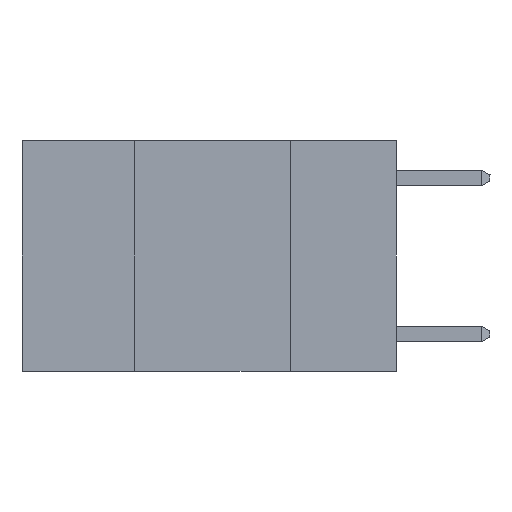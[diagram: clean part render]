
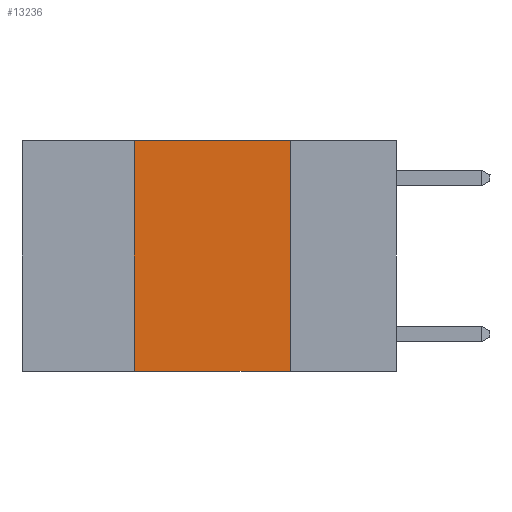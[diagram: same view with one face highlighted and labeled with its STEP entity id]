
A CAD part, left-side view. The second image highlights one B-rep face of the part: STEP entity #13236.
In plain terms, the highlighted planar face has unit normal (-1, 0, 0).
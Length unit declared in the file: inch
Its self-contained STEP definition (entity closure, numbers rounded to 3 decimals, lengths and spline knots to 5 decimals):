
#1128 = ORIENTED_EDGE ( 'NONE', *, *, #13991, .T. ) ;
#3027 = LINE ( 'NONE', #6565, #6303 ) ;
#3278 = EDGE_CURVE ( 'NONE', #15691, #15222, #6163, .T. ) ;
#3468 = PLANE ( 'NONE',  #9827 ) ;
#3547 = CARTESIAN_POINT ( 'NONE',  ( 0., 0.17, 0. ) ) ;
#3692 = LINE ( 'NONE', #3547, #11757 ) ;
#4470 = CARTESIAN_POINT ( 'NONE',  ( 0., 0.6, 0. ) ) ;
#6163 = LINE ( 'NONE', #4470, #9892 ) ;
#6303 = VECTOR ( 'NONE', #9366, 39.37008 ) ;
#6565 = CARTESIAN_POINT ( 'NONE',  ( 0., 0.6, -0.37 ) ) ;
#7215 = ORIENTED_EDGE ( 'NONE', *, *, #8718, .F. ) ;
#7657 = DIRECTION ( 'NONE',  ( 1., 0., 0. ) ) ;
#8599 = DIRECTION ( 'NONE',  ( 0., 0., 1. ) ) ;
#8718 = EDGE_CURVE ( 'NONE', #14443, #15691, #10187, .T. ) ;
#9366 = DIRECTION ( 'NONE',  ( 0., -1., 0. ) ) ;
#9404 = ORIENTED_EDGE ( 'NONE', *, *, #3278, .F. ) ;
#9827 = AXIS2_PLACEMENT_3D ( 'NONE', #14516, #7657, #17245 ) ;
#9892 = VECTOR ( 'NONE', #12747, 39.37008 ) ;
#10187 = LINE ( 'NONE', #14049, #16519 ) ;
#10795 = CARTESIAN_POINT ( 'NONE',  ( 0., 0.17, -0.37 ) ) ;
#11757 = VECTOR ( 'NONE', #13264, 39.37008 ) ;
#11807 = CARTESIAN_POINT ( 'NONE',  ( 0., 0.17, 0. ) ) ;
#12533 = EDGE_LOOP ( 'NONE', ( #17712, #9404, #7215, #1128 ) ) ;
#12604 = EDGE_CURVE ( 'NONE', #15222, #16063, #3692, .T. ) ;
#12747 = DIRECTION ( 'NONE',  ( 0., -1., 0. ) ) ;
#13236 = ADVANCED_FACE ( 'NONE', ( #14479 ), #3468, .F. ) ;
#13264 = DIRECTION ( 'NONE',  ( 0., 0., -1. ) ) ;
#13991 = EDGE_CURVE ( 'NONE', #14443, #16063, #3027, .T. ) ;
#14049 = CARTESIAN_POINT ( 'NONE',  ( 0., 0.42, 0. ) ) ;
#14443 = VERTEX_POINT ( 'NONE', #17074 ) ;
#14479 = FACE_OUTER_BOUND ( 'NONE', #12533, .T. ) ;
#14516 = CARTESIAN_POINT ( 'NONE',  ( 0., 0.6, 0. ) ) ;
#15222 = VERTEX_POINT ( 'NONE', #11807 ) ;
#15497 = CARTESIAN_POINT ( 'NONE',  ( 0., 0.42, 0. ) ) ;
#15691 = VERTEX_POINT ( 'NONE', #15497 ) ;
#16063 = VERTEX_POINT ( 'NONE', #10795 ) ;
#16519 = VECTOR ( 'NONE', #8599, 39.37008 ) ;
#17074 = CARTESIAN_POINT ( 'NONE',  ( 0., 0.42, -0.37 ) ) ;
#17245 = DIRECTION ( 'NONE',  ( 0., 0., -1. ) ) ;
#17712 = ORIENTED_EDGE ( 'NONE', *, *, #12604, .F. ) ;
